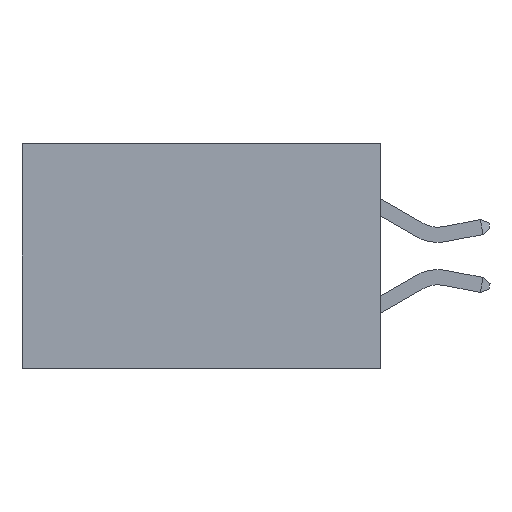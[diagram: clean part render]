
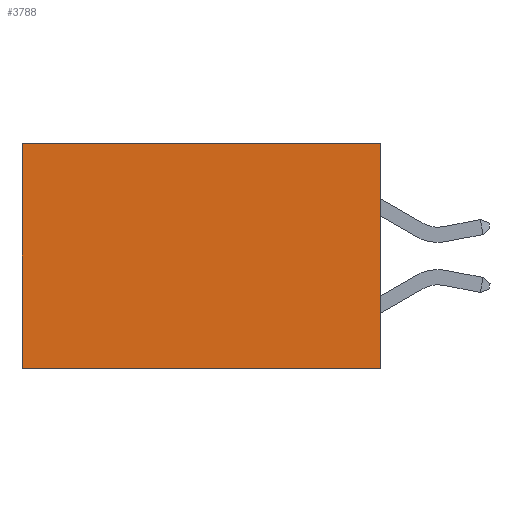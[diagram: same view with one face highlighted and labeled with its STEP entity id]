
A CAD part, left-side view. The second image highlights one B-rep face of the part: STEP entity #3788.
In plain terms, the highlighted planar face has unit normal (-1, 0, 0).
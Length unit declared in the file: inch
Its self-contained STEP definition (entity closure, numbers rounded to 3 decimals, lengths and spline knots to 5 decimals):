
#1447 = CARTESIAN_POINT ( 'NONE',  ( 0.277, 0., -0.37 ) ) ;
#1711 = CARTESIAN_POINT ( 'NONE',  ( 0.277, 0., -0.37 ) ) ;
#2061 = LINE ( 'NONE', #9223, #14160 ) ;
#2072 = ORIENTED_EDGE ( 'NONE', *, *, #19028, .F. ) ;
#2092 = VERTEX_POINT ( 'NONE', #16651 ) ;
#3106 = VERTEX_POINT ( 'NONE', #8956 ) ;
#3788 = ADVANCED_FACE ( 'NONE', ( #12706 ), #6052, .F. ) ;
#4299 = DIRECTION ( 'NONE',  ( 0., 1., 0. ) ) ;
#4582 = CARTESIAN_POINT ( 'NONE',  ( 0.277, 0.59, 0. ) ) ;
#5623 = VERTEX_POINT ( 'NONE', #4582 ) ;
#5624 = DIRECTION ( 'NONE',  ( 1., 0., 0. ) ) ;
#6052 = PLANE ( 'NONE',  #12124 ) ;
#6253 = VECTOR ( 'NONE', #4299, 39.37008 ) ;
#6332 = EDGE_LOOP ( 'NONE', ( #12074, #2072, #10449, #11144 ) ) ;
#6372 = DIRECTION ( 'NONE',  ( 0., 0., -1. ) ) ;
#7861 = DIRECTION ( 'NONE',  ( 0., 1., 0. ) ) ;
#7987 = EDGE_CURVE ( 'NONE', #5623, #16214, #2061, .T. ) ;
#8511 = DIRECTION ( 'NONE',  ( 0., 0., -1. ) ) ;
#8956 = CARTESIAN_POINT ( 'NONE',  ( 0.277, 0., -0.37 ) ) ;
#9223 = CARTESIAN_POINT ( 'NONE',  ( 0.277, 0.59, -0.37 ) ) ;
#9339 = LINE ( 'NONE', #1711, #20118 ) ;
#9719 = DIRECTION ( 'NONE',  ( 0., 0., -1. ) ) ;
#10449 = ORIENTED_EDGE ( 'NONE', *, *, #15306, .F. ) ;
#11144 = ORIENTED_EDGE ( 'NONE', *, *, #17604, .T. ) ;
#11413 = LINE ( 'NONE', #16815, #6253 ) ;
#11592 = VECTOR ( 'NONE', #7861, 39.37008 ) ;
#12074 = ORIENTED_EDGE ( 'NONE', *, *, #7987, .T. ) ;
#12124 = AXIS2_PLACEMENT_3D ( 'NONE', #14544, #5624, #6372 ) ;
#12576 = LINE ( 'NONE', #1447, #11592 ) ;
#12706 = FACE_OUTER_BOUND ( 'NONE', #6332, .T. ) ;
#14160 = VECTOR ( 'NONE', #8511, 39.37008 ) ;
#14544 = CARTESIAN_POINT ( 'NONE',  ( 0.277, 0., -0.37 ) ) ;
#15306 = EDGE_CURVE ( 'NONE', #2092, #3106, #9339, .T. ) ;
#16214 = VERTEX_POINT ( 'NONE', #19485 ) ;
#16651 = CARTESIAN_POINT ( 'NONE',  ( 0.277, 0., 0. ) ) ;
#16815 = CARTESIAN_POINT ( 'NONE',  ( 0.277, 0., 0. ) ) ;
#17604 = EDGE_CURVE ( 'NONE', #2092, #5623, #11413, .T. ) ;
#19028 = EDGE_CURVE ( 'NONE', #3106, #16214, #12576, .T. ) ;
#19485 = CARTESIAN_POINT ( 'NONE',  ( 0.277, 0.59, -0.37 ) ) ;
#20118 = VECTOR ( 'NONE', #9719, 39.37008 ) ;
